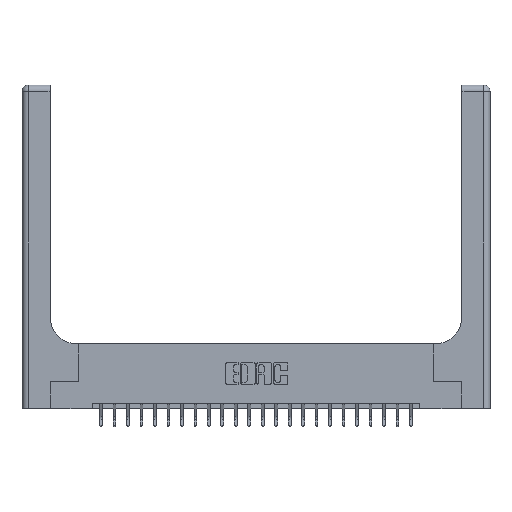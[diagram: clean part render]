
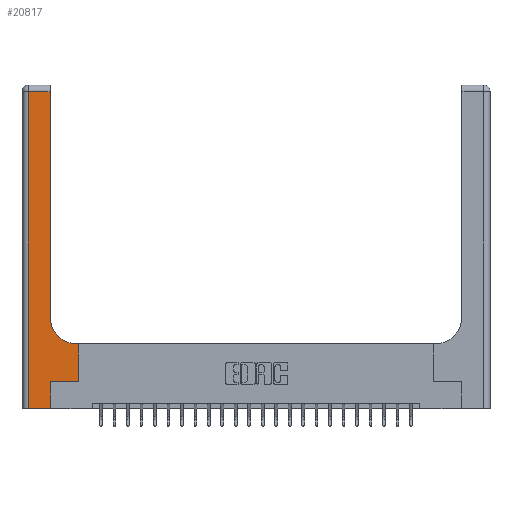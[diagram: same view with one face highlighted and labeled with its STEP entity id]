
A CAD part, top view. The second image highlights one B-rep face of the part: STEP entity #20817.
In plain terms, the highlighted planar face has unit normal (0, 0, 1).
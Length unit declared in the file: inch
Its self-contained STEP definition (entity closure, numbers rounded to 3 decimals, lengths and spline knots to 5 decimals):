
#311 = CARTESIAN_POINT ( 'NONE',  ( 0.265, 0., 0.37 ) ) ;
#331 = LINE ( 'NONE', #15102, #8581 ) ;
#776 = CARTESIAN_POINT ( 'NONE',  ( 0.528, 0.6, 0.37 ) ) ;
#1346 = DIRECTION ( 'NONE',  ( 1., 0., 0. ) ) ;
#1416 = LINE ( 'NONE', #17727, #20998 ) ;
#1499 = LINE ( 'NONE', #12652, #21921 ) ;
#1553 = EDGE_CURVE ( 'NONE', #15227, #18403, #13478, .T. ) ;
#1831 = VECTOR ( 'NONE', #6178, 39.37008 ) ;
#2093 = EDGE_CURVE ( 'NONE', #17817, #12587, #6672, .T. ) ;
#3114 = EDGE_LOOP ( 'NONE', ( #11253, #9737, #7952, #12971, #21534, #6801, #13191, #18674, #18571 ) ) ;
#4074 = CIRCLE ( 'NONE', #22974, 0.25 ) ;
#4181 = CARTESIAN_POINT ( 'NONE',  ( 0.51, 0.6, 0.37 ) ) ;
#5210 = DIRECTION ( 'NONE',  ( 1., 0., 0. ) ) ;
#5287 = DIRECTION ( 'NONE',  ( 0., 0., -1. ) ) ;
#5703 = DIRECTION ( 'NONE',  ( 0., -1., 0. ) ) ;
#6178 = DIRECTION ( 'NONE',  ( 0., 1., 0. ) ) ;
#6232 = EDGE_CURVE ( 'NONE', #14827, #10641, #4074, .T. ) ;
#6672 = LINE ( 'NONE', #7284, #1831 ) ;
#6801 = ORIENTED_EDGE ( 'NONE', *, *, #8309, .T. ) ;
#7284 = CARTESIAN_POINT ( 'NONE',  ( 0.528, 0.25, 0.37 ) ) ;
#7952 = ORIENTED_EDGE ( 'NONE', *, *, #1553, .T. ) ;
#8147 = EDGE_CURVE ( 'NONE', #17081, #15227, #16439, .T. ) ;
#8309 = EDGE_CURVE ( 'NONE', #15144, #17817, #18145, .T. ) ;
#8581 = VECTOR ( 'NONE', #15410, 39.37008 ) ;
#8647 = EDGE_CURVE ( 'NONE', #18403, #9050, #1416, .T. ) ;
#9050 = VERTEX_POINT ( 'NONE', #10096 ) ;
#9233 = CARTESIAN_POINT ( 'NONE',  ( 0.265, 0.25, 0.37 ) ) ;
#9737 = ORIENTED_EDGE ( 'NONE', *, *, #8147, .T. ) ;
#10086 = EDGE_CURVE ( 'NONE', #9050, #15144, #15259, .T. ) ;
#10096 = CARTESIAN_POINT ( 'NONE',  ( 0.265, 0., 0.37 ) ) ;
#10641 = VERTEX_POINT ( 'NONE', #20462 ) ;
#10664 = DIRECTION ( 'NONE',  ( -1., 0., 0. ) ) ;
#10813 = PLANE ( 'NONE',  #21356 ) ;
#11144 = CARTESIAN_POINT ( 'NONE',  ( 0.26, 2.94, 0.37 ) ) ;
#11253 = ORIENTED_EDGE ( 'NONE', *, *, #22367, .T. ) ;
#11649 = VECTOR ( 'NONE', #16514, 39.37008 ) ;
#11690 = CARTESIAN_POINT ( 'NONE',  ( 0.528, 0.25, 0.37 ) ) ;
#12587 = VERTEX_POINT ( 'NONE', #776 ) ;
#12652 = CARTESIAN_POINT ( 'NONE',  ( 0.26, 3., 0.37 ) ) ;
#12971 = ORIENTED_EDGE ( 'NONE', *, *, #8647, .T. ) ;
#13191 = ORIENTED_EDGE ( 'NONE', *, *, #2093, .T. ) ;
#13478 = LINE ( 'NONE', #15981, #19456 ) ;
#14394 = DIRECTION ( 'NONE',  ( 0., 1., 0. ) ) ;
#14827 = VERTEX_POINT ( 'NONE', #4181 ) ;
#15102 = CARTESIAN_POINT ( 'NONE',  ( 0.26, 0.6, 0.37 ) ) ;
#15140 = CARTESIAN_POINT ( 'NONE',  ( 0.06, 0., 0.37 ) ) ;
#15144 = VERTEX_POINT ( 'NONE', #9233 ) ;
#15227 = VERTEX_POINT ( 'NONE', #20275 ) ;
#15259 = LINE ( 'NONE', #311, #20699 ) ;
#15410 = DIRECTION ( 'NONE',  ( -1., 0., 0. ) ) ;
#15521 = CARTESIAN_POINT ( 'NONE',  ( 0.51, 0.85, 0.37 ) ) ;
#15981 = CARTESIAN_POINT ( 'NONE',  ( 0.06, 3., 0.37 ) ) ;
#16115 = CARTESIAN_POINT ( 'NONE',  ( 0., 3., 0.37 ) ) ;
#16439 = LINE ( 'NONE', #21940, #11649 ) ;
#16514 = DIRECTION ( 'NONE',  ( -1., 0., 0. ) ) ;
#17081 = VERTEX_POINT ( 'NONE', #11144 ) ;
#17586 = VECTOR ( 'NONE', #5210, 39.37008 ) ;
#17727 = CARTESIAN_POINT ( 'NONE',  ( 0., 0., 0.37 ) ) ;
#17817 = VERTEX_POINT ( 'NONE', #11690 ) ;
#18145 = LINE ( 'NONE', #18951, #17586 ) ;
#18403 = VERTEX_POINT ( 'NONE', #15140 ) ;
#18571 = ORIENTED_EDGE ( 'NONE', *, *, #6232, .T. ) ;
#18674 = ORIENTED_EDGE ( 'NONE', *, *, #22615, .T. ) ;
#18951 = CARTESIAN_POINT ( 'NONE',  ( 0.265, 0.25, 0.37 ) ) ;
#19456 = VECTOR ( 'NONE', #5703, 39.37008 ) ;
#20086 = DIRECTION ( 'NONE',  ( 0., 1., 0. ) ) ;
#20275 = CARTESIAN_POINT ( 'NONE',  ( 0.06, 2.94, 0.37 ) ) ;
#20462 = CARTESIAN_POINT ( 'NONE',  ( 0.26, 0.85, 0.37 ) ) ;
#20699 = VECTOR ( 'NONE', #20086, 39.37008 ) ;
#20817 = ADVANCED_FACE ( 'NONE', ( #23144 ), #10813, .F. ) ;
#20998 = VECTOR ( 'NONE', #23378, 39.37008 ) ;
#21024 = DIRECTION ( 'NONE',  ( 0., 0., -1. ) ) ;
#21356 = AXIS2_PLACEMENT_3D ( 'NONE', #16115, #5287, #10664 ) ;
#21534 = ORIENTED_EDGE ( 'NONE', *, *, #10086, .T. ) ;
#21921 = VECTOR ( 'NONE', #14394, 39.37008 ) ;
#21940 = CARTESIAN_POINT ( 'NONE',  ( 0., 2.94, 0.37 ) ) ;
#22367 = EDGE_CURVE ( 'NONE', #10641, #17081, #1499, .T. ) ;
#22615 = EDGE_CURVE ( 'NONE', #12587, #14827, #331, .T. ) ;
#22974 = AXIS2_PLACEMENT_3D ( 'NONE', #15521, #21024, #1346 ) ;
#23144 = FACE_OUTER_BOUND ( 'NONE', #3114, .T. ) ;
#23378 = DIRECTION ( 'NONE',  ( 1., 0., 0. ) ) ;
